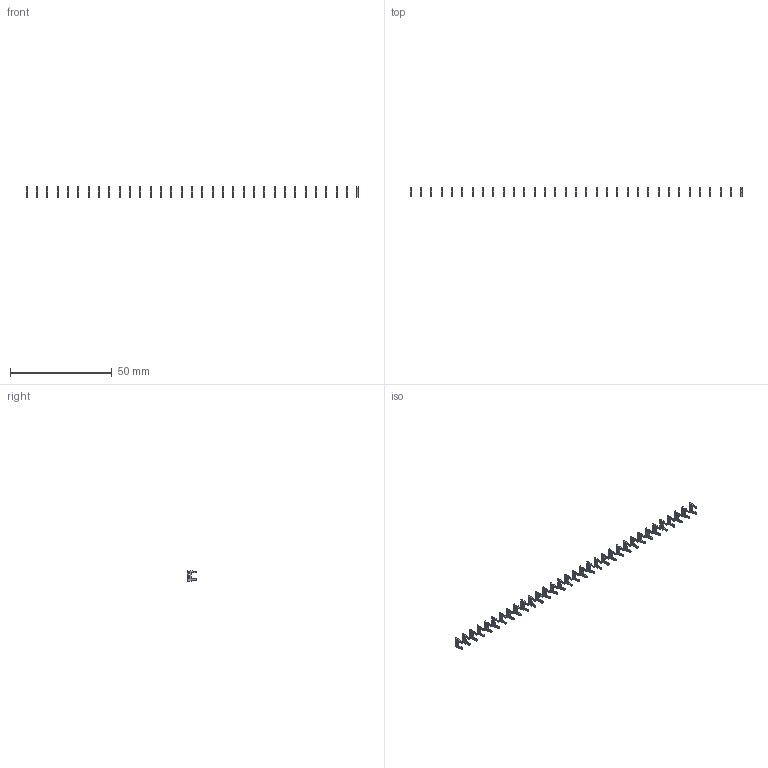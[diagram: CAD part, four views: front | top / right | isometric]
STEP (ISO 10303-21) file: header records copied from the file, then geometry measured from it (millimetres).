
FILE_DESCRIPTION (( 'STEP AP203' ), '1' );
FILE_NAME ('105-033-208-200.STEP', '2020-04-07T23:36:51', ( '' ), ( '' ), 'SwSTEP 2.0', 'SolidWorks 2016', '' );
FILE_SCHEMA (( 'CONFIG_CONTROL_DESIGN' ));
Length unit declared in the file: inch
Products named in the file (2): 105-033-208-200; 100-290-001_100-290-208
Assembly tree (33 placements, depth 2):
  105-033-208-200
    100-290-001_100-290-208  x33
Bounding box: 163.07 x 4.83 x 5.17 mm (x, y, z)
Volume: 227.1 mm3; surface area: 1402.4 mm2
Topology: 33 solids, 33 shells, 825 faces, 2277 edges, 1518 vertices
Faces by surface type: plane 726, cylinder 99
Entity records: 2013 total; most frequent: DIRECTION 197, CARTESIAN_POINT 176, ORIENTED_EDGE 138, DATE_AND_TIME 76, COORDINATED_UNIVERSAL_TIME_OFFSET 76, CALENDAR_DATE 76, LOCAL_TIME 76, EDGE_CURVE 69
